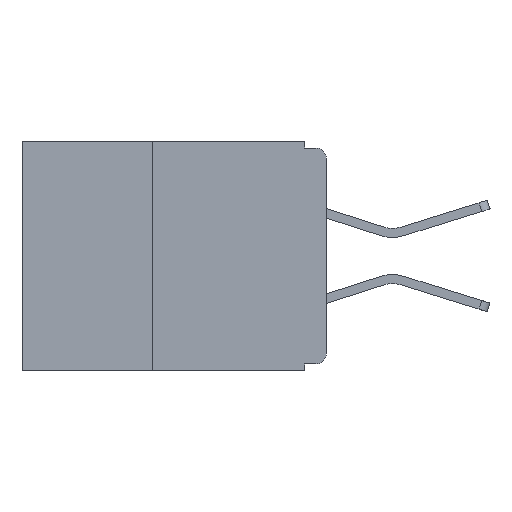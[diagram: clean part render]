
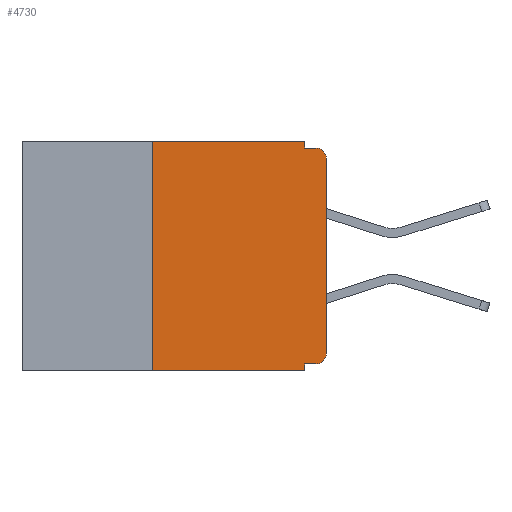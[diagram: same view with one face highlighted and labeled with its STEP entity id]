
A CAD part, left-side view. The second image highlights one B-rep face of the part: STEP entity #4730.
In plain terms, the highlighted planar face has unit normal (-1, 0, 0).
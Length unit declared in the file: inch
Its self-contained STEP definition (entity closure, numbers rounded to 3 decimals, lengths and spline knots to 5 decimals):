
#9 = CARTESIAN_POINT ( 'NONE',  ( 0., 0.015, -0.305 ) ) ;
#947 = CARTESIAN_POINT ( 'NONE',  ( 0., 0.015, -0.025 ) ) ;
#1641 = CARTESIAN_POINT ( 'NONE',  ( 0., 0.25, 0. ) ) ;
#2265 = ORIENTED_EDGE ( 'NONE', *, *, #27425, .F. ) ;
#2421 = FACE_OUTER_BOUND ( 'NONE', #30332, .T. ) ;
#2492 = DIRECTION ( 'NONE',  ( 0., 0., -1. ) ) ;
#2562 = VECTOR ( 'NONE', #8348, 39.37008 ) ;
#3033 = CARTESIAN_POINT ( 'NONE',  ( 0., 0.031, 0. ) ) ;
#3442 = DIRECTION ( 'NONE',  ( 0., 0., -1. ) ) ;
#4730 = ADVANCED_FACE ( 'NONE', ( #2421 ), #15451, .F. ) ;
#6266 = VERTEX_POINT ( 'NONE', #7543 ) ;
#6348 = VERTEX_POINT ( 'NONE', #26617 ) ;
#7457 = DIRECTION ( 'NONE',  ( 0., 0., -1. ) ) ;
#7543 = CARTESIAN_POINT ( 'NONE',  ( 0., 0.031, -0.32 ) ) ;
#7867 = DIRECTION ( 'NONE',  ( 0., -1., 0. ) ) ;
#7959 = EDGE_CURVE ( 'NONE', #29844, #21241, #29290, .T. ) ;
#8077 = DIRECTION ( 'NONE',  ( 0., 1., 0. ) ) ;
#8253 = VECTOR ( 'NONE', #20867, 39.37008 ) ;
#8348 = DIRECTION ( 'NONE',  ( 0., 0., -1. ) ) ;
#8530 = VERTEX_POINT ( 'NONE', #23385 ) ;
#8550 = VECTOR ( 'NONE', #12893, 39.37008 ) ;
#8609 = EDGE_CURVE ( 'NONE', #12130, #16125, #23893, .T. ) ;
#8679 = ORIENTED_EDGE ( 'NONE', *, *, #7959, .F. ) ;
#8946 = ORIENTED_EDGE ( 'NONE', *, *, #19655, .T. ) ;
#9072 = CIRCLE ( 'NONE', #10846, 0.015 ) ;
#9285 = ORIENTED_EDGE ( 'NONE', *, *, #15879, .F. ) ;
#9905 = VECTOR ( 'NONE', #19027, 39.37008 ) ;
#10207 = CARTESIAN_POINT ( 'NONE',  ( 0., 0.437, -0.33 ) ) ;
#10231 = CARTESIAN_POINT ( 'NONE',  ( 0., 0.031, -0.33 ) ) ;
#10846 = AXIS2_PLACEMENT_3D ( 'NONE', #947, #17625, #3442 ) ;
#11081 = LINE ( 'NONE', #12091, #16637 ) ;
#11377 = CARTESIAN_POINT ( 'NONE',  ( 0., 0.015, -0.01 ) ) ;
#11382 = CARTESIAN_POINT ( 'NONE',  ( 0., 0., -0.01 ) ) ;
#11468 = LINE ( 'NONE', #19008, #28688 ) ;
#12091 = CARTESIAN_POINT ( 'NONE',  ( 0., 0.031, -0.33 ) ) ;
#12130 = VERTEX_POINT ( 'NONE', #21603 ) ;
#12302 = ORIENTED_EDGE ( 'NONE', *, *, #23281, .F. ) ;
#12312 = AXIS2_PLACEMENT_3D ( 'NONE', #15786, #14825, #14748 ) ;
#12475 = ORIENTED_EDGE ( 'NONE', *, *, #8609, .T. ) ;
#12723 = VERTEX_POINT ( 'NONE', #10231 ) ;
#12893 = DIRECTION ( 'NONE',  ( 0., -1., 0. ) ) ;
#14190 = AXIS2_PLACEMENT_3D ( 'NONE', #9, #16715, #2492 ) ;
#14342 = EDGE_CURVE ( 'NONE', #8530, #28998, #14538, .T. ) ;
#14538 = LINE ( 'NONE', #11382, #8253 ) ;
#14748 = DIRECTION ( 'NONE',  ( 0., 0., -1. ) ) ;
#14825 = DIRECTION ( 'NONE',  ( 1., 0., 0. ) ) ;
#14840 = ORIENTED_EDGE ( 'NONE', *, *, #14342, .F. ) ;
#15112 = CARTESIAN_POINT ( 'NONE',  ( 0., 0., -0.32 ) ) ;
#15243 = VERTEX_POINT ( 'NONE', #3033 ) ;
#15451 = PLANE ( 'NONE',  #12312 ) ;
#15786 = CARTESIAN_POINT ( 'NONE',  ( 0., 0.437, 0. ) ) ;
#15879 = EDGE_CURVE ( 'NONE', #15243, #8530, #21446, .T. ) ;
#16125 = VERTEX_POINT ( 'NONE', #30074 ) ;
#16637 = VECTOR ( 'NONE', #7457, 39.37008 ) ;
#16649 = CARTESIAN_POINT ( 'NONE',  ( 0., 0.25, -0.33 ) ) ;
#16715 = DIRECTION ( 'NONE',  ( -1., 0., 0. ) ) ;
#17457 = DIRECTION ( 'NONE',  ( 0., 0., 1. ) ) ;
#17625 = DIRECTION ( 'NONE',  ( -1., 0., 0. ) ) ;
#17938 = VECTOR ( 'NONE', #7867, 39.37008 ) ;
#19008 = CARTESIAN_POINT ( 'NONE',  ( 0., 0., 0. ) ) ;
#19027 = DIRECTION ( 'NONE',  ( 0., 0., 1. ) ) ;
#19305 = CARTESIAN_POINT ( 'NONE',  ( 0., 0.25, -0.33 ) ) ;
#19388 = ORIENTED_EDGE ( 'NONE', *, *, #23192, .T. ) ;
#19655 = EDGE_CURVE ( 'NONE', #6348, #28998, #9072, .T. ) ;
#20014 = CARTESIAN_POINT ( 'NONE',  ( 0., 0.437, 0. ) ) ;
#20088 = CARTESIAN_POINT ( 'NONE',  ( 0., 0.031, 0. ) ) ;
#20867 = DIRECTION ( 'NONE',  ( 0., -1., 0. ) ) ;
#21052 = LINE ( 'NONE', #20014, #8550 ) ;
#21241 = VERTEX_POINT ( 'NONE', #1641 ) ;
#21446 = LINE ( 'NONE', #20088, #2562 ) ;
#21603 = CARTESIAN_POINT ( 'NONE',  ( 0., 0.015, -0.32 ) ) ;
#22708 = VECTOR ( 'NONE', #8077, 39.37008 ) ;
#22754 = EDGE_CURVE ( 'NONE', #6266, #12723, #11081, .T. ) ;
#23192 = EDGE_CURVE ( 'NONE', #16125, #6348, #11468, .T. ) ;
#23281 = EDGE_CURVE ( 'NONE', #21241, #15243, #21052, .T. ) ;
#23385 = CARTESIAN_POINT ( 'NONE',  ( 0., 0.031, -0.01 ) ) ;
#23436 = LINE ( 'NONE', #15112, #22708 ) ;
#23893 = CIRCLE ( 'NONE', #14190, 0.015 ) ;
#24138 = LINE ( 'NONE', #10207, #17938 ) ;
#26617 = CARTESIAN_POINT ( 'NONE',  ( 0., 0., -0.025 ) ) ;
#27387 = EDGE_CURVE ( 'NONE', #29844, #12723, #24138, .T. ) ;
#27425 = EDGE_CURVE ( 'NONE', #12130, #6266, #23436, .T. ) ;
#28479 = ORIENTED_EDGE ( 'NONE', *, *, #22754, .F. ) ;
#28688 = VECTOR ( 'NONE', #17457, 39.37008 ) ;
#28998 = VERTEX_POINT ( 'NONE', #11377 ) ;
#29290 = LINE ( 'NONE', #16649, #9905 ) ;
#29844 = VERTEX_POINT ( 'NONE', #19305 ) ;
#30074 = CARTESIAN_POINT ( 'NONE',  ( 0., 0., -0.305 ) ) ;
#30199 = ORIENTED_EDGE ( 'NONE', *, *, #27387, .T. ) ;
#30332 = EDGE_LOOP ( 'NONE', ( #19388, #8946, #14840, #9285, #12302, #8679, #30199, #28479, #2265, #12475 ) ) ;
